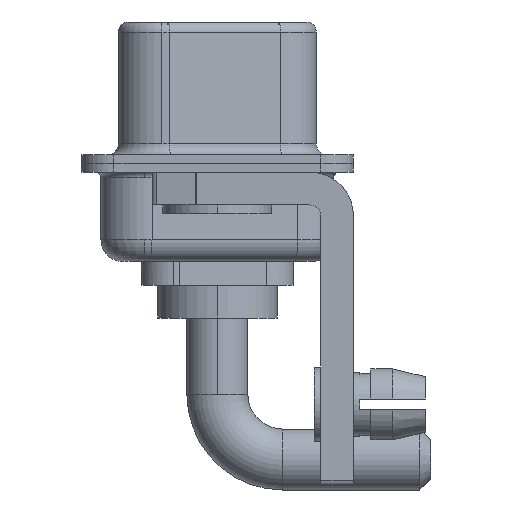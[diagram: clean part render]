
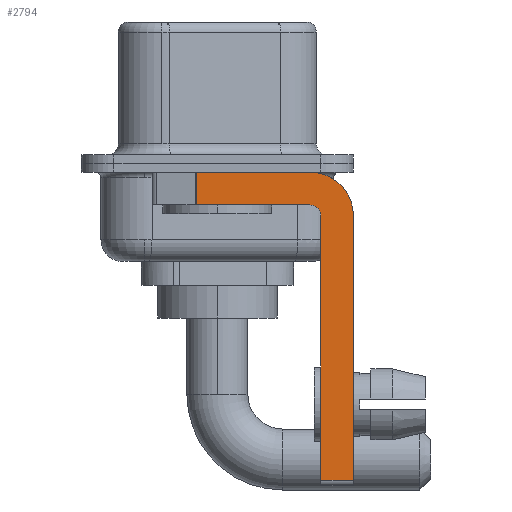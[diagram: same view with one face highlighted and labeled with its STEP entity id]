
A CAD part, left-side view. The second image highlights one B-rep face of the part: STEP entity #2794.
In plain terms, the highlighted planar face has unit normal (-1, 0, 0).
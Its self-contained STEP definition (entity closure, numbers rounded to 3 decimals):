
#271 = VECTOR ( 'NONE', #9454, 1000. ) ;
#388 = EDGE_CURVE ( 'NONE', #1454, #10461, #12676, .T. ) ;
#427 = LINE ( 'NONE', #5932, #14232 ) ;
#612 = DIRECTION ( 'NONE',  ( 0., -1., 0. ) ) ;
#728 = VERTEX_POINT ( 'NONE', #6693 ) ;
#979 = FACE_OUTER_BOUND ( 'NONE', #12390, .T. ) ;
#1061 = CARTESIAN_POINT ( 'NONE',  ( -2.9, 0.978, -1.9 ) ) ;
#1454 = VERTEX_POINT ( 'NONE', #9972 ) ;
#1565 = CARTESIAN_POINT ( 'NONE',  ( -2.9, -4.25, -1.9 ) ) ;
#2067 = EDGE_CURVE ( 'NONE', #728, #17558, #17340, .T. ) ;
#2113 = AXIS2_PLACEMENT_3D ( 'NONE', #2562, #2649, #9664 ) ;
#2174 = CARTESIAN_POINT ( 'NONE',  ( -2.9, -6.25, -2.4 ) ) ;
#2229 = VERTEX_POINT ( 'NONE', #9030 ) ;
#2489 = EDGE_CURVE ( 'NONE', #12524, #2887, #16125, .T. ) ;
#2562 = CARTESIAN_POINT ( 'NONE',  ( -2.9, -4.25, -2.4 ) ) ;
#2649 = DIRECTION ( 'NONE',  ( -1., 0., 0. ) ) ;
#2794 = ADVANCED_FACE ( 'NONE', ( #979 ), #16830, .F. ) ;
#2887 = VERTEX_POINT ( 'NONE', #3108 ) ;
#2972 = VECTOR ( 'NONE', #9867, 1000. ) ;
#3108 = CARTESIAN_POINT ( 'NONE',  ( -2.9, -6.25, -2.4 ) ) ;
#3433 = CARTESIAN_POINT ( 'NONE',  ( -2.9, -4.75, -14.8 ) ) ;
#4065 = CARTESIAN_POINT ( 'NONE',  ( -2.9, -4.25, -0.4 ) ) ;
#4176 = VECTOR ( 'NONE', #16372, 1000. ) ;
#4281 = ORIENTED_EDGE ( 'NONE', *, *, #2067, .F. ) ;
#4352 = CARTESIAN_POINT ( 'NONE',  ( -2.9, -4.25, -2.4 ) ) ;
#4451 = ORIENTED_EDGE ( 'NONE', *, *, #17180, .F. ) ;
#5197 = ORIENTED_EDGE ( 'NONE', *, *, #2489, .F. ) ;
#5411 = CARTESIAN_POINT ( 'NONE',  ( -2.9, -6.25, -14.55 ) ) ;
#5932 = CARTESIAN_POINT ( 'NONE',  ( -2.9, 3., -0.4 ) ) ;
#6560 = VECTOR ( 'NONE', #14347, 1000. ) ;
#6666 = CARTESIAN_POINT ( 'NONE',  ( -2.9, -4.25, -2.4 ) ) ;
#6693 = CARTESIAN_POINT ( 'NONE',  ( -2.9, -4.25, -1.9 ) ) ;
#6752 = DIRECTION ( 'NONE',  ( 1., 0., 0. ) ) ;
#7149 = DIRECTION ( 'NONE',  ( 0., 0., -1. ) ) ;
#7874 = LINE ( 'NONE', #2174, #271 ) ;
#8037 = CARTESIAN_POINT ( 'NONE',  ( -2.9, 0.978, -0.4 ) ) ;
#8408 = EDGE_CURVE ( 'NONE', #2887, #10461, #7874, .T. ) ;
#8670 = AXIS2_PLACEMENT_3D ( 'NONE', #4352, #11521, #7149 ) ;
#9030 = CARTESIAN_POINT ( 'NONE',  ( -2.9, -4.75, -2.4 ) ) ;
#9454 = DIRECTION ( 'NONE',  ( 0., 0., -1. ) ) ;
#9502 = EDGE_CURVE ( 'NONE', #1454, #2229, #16233, .T. ) ;
#9664 = DIRECTION ( 'NONE',  ( 0., 0., 1. ) ) ;
#9867 = DIRECTION ( 'NONE',  ( 0., -1., 0. ) ) ;
#9972 = CARTESIAN_POINT ( 'NONE',  ( -2.9, -4.75, -14.55 ) ) ;
#10142 = CARTESIAN_POINT ( 'NONE',  ( -2.9, -4.25, -14.55 ) ) ;
#10461 = VERTEX_POINT ( 'NONE', #5411 ) ;
#11521 = DIRECTION ( 'NONE',  ( 1., 0., 0. ) ) ;
#11787 = ORIENTED_EDGE ( 'NONE', *, *, #388, .T. ) ;
#12390 = EDGE_LOOP ( 'NONE', ( #16173, #13033, #4281, #4451, #14345, #11787, #13041, #5197 ) ) ;
#12524 = VERTEX_POINT ( 'NONE', #4065 ) ;
#12676 = LINE ( 'NONE', #10142, #2972 ) ;
#13033 = ORIENTED_EDGE ( 'NONE', *, *, #16119, .T. ) ;
#13041 = ORIENTED_EDGE ( 'NONE', *, *, #8408, .F. ) ;
#13562 = CARTESIAN_POINT ( 'NONE',  ( -2.9, 0.978, -1.9 ) ) ;
#13838 = LINE ( 'NONE', #13562, #4176 ) ;
#14178 = EDGE_CURVE ( 'NONE', #16690, #12524, #427, .T. ) ;
#14232 = VECTOR ( 'NONE', #612, 1000. ) ;
#14345 = ORIENTED_EDGE ( 'NONE', *, *, #9502, .F. ) ;
#14347 = DIRECTION ( 'NONE',  ( 0., 1., 0. ) ) ;
#14827 = DIRECTION ( 'NONE',  ( 0., 0., 1. ) ) ;
#16119 = EDGE_CURVE ( 'NONE', #16690, #17558, #13838, .T. ) ;
#16125 = CIRCLE ( 'NONE', #8670, 2. ) ;
#16173 = ORIENTED_EDGE ( 'NONE', *, *, #14178, .F. ) ;
#16233 = LINE ( 'NONE', #3433, #18042 ) ;
#16372 = DIRECTION ( 'NONE',  ( 0., 0., -1. ) ) ;
#16690 = VERTEX_POINT ( 'NONE', #8037 ) ;
#16830 = PLANE ( 'NONE',  #17909 ) ;
#17180 = EDGE_CURVE ( 'NONE', #2229, #728, #17626, .T. ) ;
#17340 = LINE ( 'NONE', #1565, #6560 ) ;
#17558 = VERTEX_POINT ( 'NONE', #1061 ) ;
#17626 = CIRCLE ( 'NONE', #2113, 0.5 ) ;
#17909 = AXIS2_PLACEMENT_3D ( 'NONE', #6666, #6752, #18067 ) ;
#18042 = VECTOR ( 'NONE', #14827, 1000. ) ;
#18067 = DIRECTION ( 'NONE',  ( 0., 0., -1. ) ) ;
